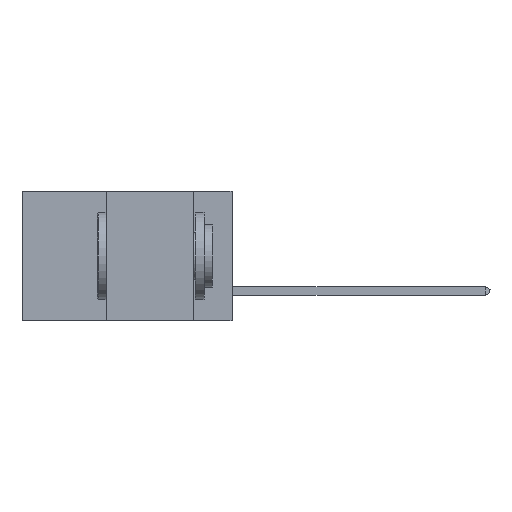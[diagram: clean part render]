
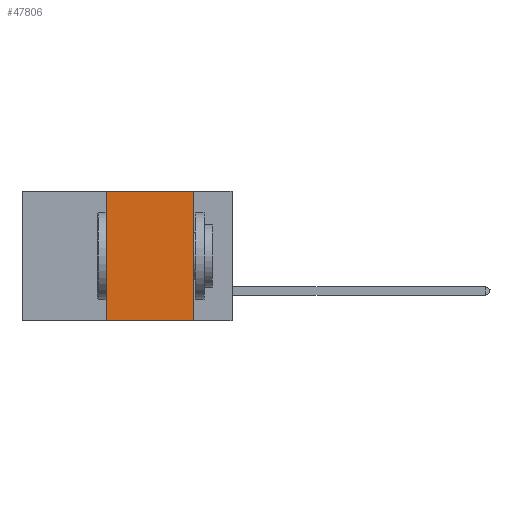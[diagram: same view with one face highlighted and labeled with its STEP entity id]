
A CAD part, left-side view. The second image highlights one B-rep face of the part: STEP entity #47806.
In plain terms, the highlighted planar face has unit normal (-1, 0, 0).
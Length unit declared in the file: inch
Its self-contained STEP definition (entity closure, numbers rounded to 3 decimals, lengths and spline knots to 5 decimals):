
#3096 = LINE ( 'NONE', #11170, #23762 ) ;
#5229 = CARTESIAN_POINT ( 'NONE',  ( 0., 0.36, 0. ) ) ;
#5345 = CARTESIAN_POINT ( 'NONE',  ( 0., 0.6, 0. ) ) ;
#5645 = VECTOR ( 'NONE', #12446, 39.37008 ) ;
#6370 = ORIENTED_EDGE ( 'NONE', *, *, #35726, .F. ) ;
#7258 = VERTEX_POINT ( 'NONE', #21880 ) ;
#7794 = CARTESIAN_POINT ( 'NONE',  ( 0., 0.6, 0. ) ) ;
#10699 = CARTESIAN_POINT ( 'NONE',  ( 0., 0.36, -0.37 ) ) ;
#11170 = CARTESIAN_POINT ( 'NONE',  ( 0., 0.11, 0. ) ) ;
#12446 = DIRECTION ( 'NONE',  ( 0., 0., 1. ) ) ;
#12501 = PLANE ( 'NONE',  #43229 ) ;
#14399 = EDGE_CURVE ( 'NONE', #29482, #7258, #28756, .T. ) ;
#15113 = ORIENTED_EDGE ( 'NONE', *, *, #14399, .F. ) ;
#16661 = LINE ( 'NONE', #26175, #43979 ) ;
#21880 = CARTESIAN_POINT ( 'NONE',  ( 0., 0.11, 0. ) ) ;
#22378 = DIRECTION ( 'NONE',  ( 0., 0., -1. ) ) ;
#23504 = VERTEX_POINT ( 'NONE', #10699 ) ;
#23762 = VECTOR ( 'NONE', #22378, 39.37008 ) ;
#26175 = CARTESIAN_POINT ( 'NONE',  ( 0., 0.6, -0.37 ) ) ;
#26635 = DIRECTION ( 'NONE',  ( 0., -1., 0. ) ) ;
#27453 = CARTESIAN_POINT ( 'NONE',  ( 0., 0.11, -0.37 ) ) ;
#28756 = LINE ( 'NONE', #7794, #42112 ) ;
#29482 = VERTEX_POINT ( 'NONE', #5229 ) ;
#31630 = EDGE_CURVE ( 'NONE', #23504, #47680, #16661, .T. ) ;
#32981 = LINE ( 'NONE', #44176, #5645 ) ;
#35726 = EDGE_CURVE ( 'NONE', #7258, #47680, #3096, .T. ) ;
#37914 = DIRECTION ( 'NONE',  ( 0., -1., 0. ) ) ;
#39837 = DIRECTION ( 'NONE',  ( 1., 0., 0. ) ) ;
#42112 = VECTOR ( 'NONE', #26635, 39.37008 ) ;
#43229 = AXIS2_PLACEMENT_3D ( 'NONE', #5345, #39837, #47983 ) ;
#43627 = FACE_OUTER_BOUND ( 'NONE', #46256, .T. ) ;
#43979 = VECTOR ( 'NONE', #37914, 39.37008 ) ;
#44176 = CARTESIAN_POINT ( 'NONE',  ( 0., 0.36, 0. ) ) ;
#45806 = EDGE_CURVE ( 'NONE', #23504, #29482, #32981, .T. ) ;
#46192 = ORIENTED_EDGE ( 'NONE', *, *, #31630, .T. ) ;
#46256 = EDGE_LOOP ( 'NONE', ( #6370, #15113, #49328, #46192 ) ) ;
#47680 = VERTEX_POINT ( 'NONE', #27453 ) ;
#47806 = ADVANCED_FACE ( 'NONE', ( #43627 ), #12501, .F. ) ;
#47983 = DIRECTION ( 'NONE',  ( 0., 0., -1. ) ) ;
#49328 = ORIENTED_EDGE ( 'NONE', *, *, #45806, .F. ) ;
